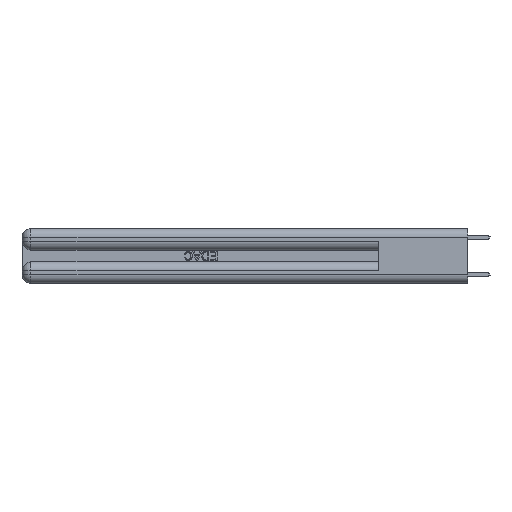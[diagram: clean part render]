
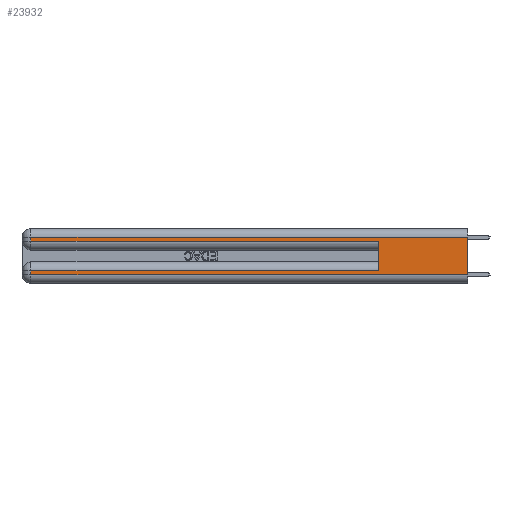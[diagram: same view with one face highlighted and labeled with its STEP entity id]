
A CAD part, left-side view. The second image highlights one B-rep face of the part: STEP entity #23932.
In plain terms, the highlighted planar face has unit normal (-1, 0, 0).
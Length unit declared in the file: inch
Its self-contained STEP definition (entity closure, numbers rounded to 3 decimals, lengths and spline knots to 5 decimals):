
#263 = LINE ( 'NONE', #33791, #25701 ) ;
#1139 = DIRECTION ( 'NONE',  ( 1., 0., 0. ) ) ;
#1954 = DIRECTION ( 'NONE',  ( 0., 0., -1. ) ) ;
#2128 = LINE ( 'NONE', #21906, #21447 ) ;
#2943 = DIRECTION ( 'NONE',  ( 0., 1., 0. ) ) ;
#3316 = VERTEX_POINT ( 'NONE', #34094 ) ;
#3340 = CARTESIAN_POINT ( 'NONE',  ( 0., 0., 0.37 ) ) ;
#3345 = VECTOR ( 'NONE', #18970, 39.37008 ) ;
#4038 = EDGE_CURVE ( 'NONE', #14277, #7153, #32106, .T. ) ;
#4164 = EDGE_CURVE ( 'NONE', #3316, #26474, #19611, .T. ) ;
#4542 = VECTOR ( 'NONE', #11597, 39.37008 ) ;
#4873 = CARTESIAN_POINT ( 'NONE',  ( 0., 2.94, 0.285 ) ) ;
#6800 = LINE ( 'NONE', #12837, #33855 ) ;
#7153 = VERTEX_POINT ( 'NONE', #12685 ) ;
#7225 = CARTESIAN_POINT ( 'NONE',  ( 0., 0., 0.085 ) ) ;
#8995 = ORIENTED_EDGE ( 'NONE', *, *, #10728, .T. ) ;
#9188 = VECTOR ( 'NONE', #35617, 39.37008 ) ;
#9305 = EDGE_LOOP ( 'NONE', ( #20092, #23945, #29942, #35041, #35452, #8995, #16218, #33614 ) ) ;
#10543 = CARTESIAN_POINT ( 'NONE',  ( 0., 0., 0.37 ) ) ;
#10728 = EDGE_CURVE ( 'NONE', #11101, #10753, #18948, .T. ) ;
#10753 = VERTEX_POINT ( 'NONE', #21346 ) ;
#10976 = EDGE_CURVE ( 'NONE', #26474, #23156, #17274, .T. ) ;
#11101 = VERTEX_POINT ( 'NONE', #29721 ) ;
#11597 = DIRECTION ( 'NONE',  ( 0., 0., -1. ) ) ;
#12053 = VERTEX_POINT ( 'NONE', #16623 ) ;
#12293 = FACE_OUTER_BOUND ( 'NONE', #9305, .T. ) ;
#12685 = CARTESIAN_POINT ( 'NONE',  ( 0., 0., 0.06 ) ) ;
#12837 = CARTESIAN_POINT ( 'NONE',  ( 0., 0., 0.285 ) ) ;
#12854 = CARTESIAN_POINT ( 'NONE',  ( 0., 0., 0.06 ) ) ;
#13350 = AXIS2_PLACEMENT_3D ( 'NONE', #3340, #1139, #33747 ) ;
#14277 = VERTEX_POINT ( 'NONE', #30823 ) ;
#14727 = DIRECTION ( 'NONE',  ( 0., 0., 1. ) ) ;
#15445 = VECTOR ( 'NONE', #2943, 39.37008 ) ;
#16042 = CARTESIAN_POINT ( 'NONE',  ( 0., 2.94, 0.31 ) ) ;
#16218 = ORIENTED_EDGE ( 'NONE', *, *, #32155, .T. ) ;
#16623 = CARTESIAN_POINT ( 'NONE',  ( 0., 0.6, 0.285 ) ) ;
#17274 = LINE ( 'NONE', #23135, #4542 ) ;
#18948 = LINE ( 'NONE', #7225, #9188 ) ;
#18970 = DIRECTION ( 'NONE',  ( 0., 0., -1. ) ) ;
#19611 = LINE ( 'NONE', #30781, #15445 ) ;
#20092 = ORIENTED_EDGE ( 'NONE', *, *, #31036, .F. ) ;
#21346 = CARTESIAN_POINT ( 'NONE',  ( 0., 2.94, 0.085 ) ) ;
#21447 = VECTOR ( 'NONE', #1954, 39.37008 ) ;
#21891 = VECTOR ( 'NONE', #27150, 39.37008 ) ;
#21906 = CARTESIAN_POINT ( 'NONE',  ( 0., 2.94, 0.37 ) ) ;
#23135 = CARTESIAN_POINT ( 'NONE',  ( 0., 2.94, 0.37 ) ) ;
#23156 = VERTEX_POINT ( 'NONE', #4873 ) ;
#23932 = ADVANCED_FACE ( 'NONE', ( #12293 ), #28815, .F. ) ;
#23945 = ORIENTED_EDGE ( 'NONE', *, *, #4164, .T. ) ;
#24023 = DIRECTION ( 'NONE',  ( 0., -1., 0. ) ) ;
#24066 = EDGE_CURVE ( 'NONE', #23156, #12053, #6800, .T. ) ;
#24827 = EDGE_CURVE ( 'NONE', #11101, #12053, #263, .T. ) ;
#25701 = VECTOR ( 'NONE', #14727, 39.37008 ) ;
#26474 = VERTEX_POINT ( 'NONE', #16042 ) ;
#27150 = DIRECTION ( 'NONE',  ( 0., -1., 0. ) ) ;
#28815 = PLANE ( 'NONE',  #13350 ) ;
#29427 = LINE ( 'NONE', #10543, #3345 ) ;
#29721 = CARTESIAN_POINT ( 'NONE',  ( 0., 0.6, 0.085 ) ) ;
#29942 = ORIENTED_EDGE ( 'NONE', *, *, #10976, .T. ) ;
#30781 = CARTESIAN_POINT ( 'NONE',  ( 0., 0., 0.31 ) ) ;
#30823 = CARTESIAN_POINT ( 'NONE',  ( 0., 2.94, 0.06 ) ) ;
#31036 = EDGE_CURVE ( 'NONE', #3316, #7153, #29427, .T. ) ;
#32106 = LINE ( 'NONE', #12854, #21891 ) ;
#32155 = EDGE_CURVE ( 'NONE', #10753, #14277, #2128, .T. ) ;
#33614 = ORIENTED_EDGE ( 'NONE', *, *, #4038, .T. ) ;
#33747 = DIRECTION ( 'NONE',  ( 0., 0., -1. ) ) ;
#33791 = CARTESIAN_POINT ( 'NONE',  ( 0., 0.6, 0.145 ) ) ;
#33855 = VECTOR ( 'NONE', #24023, 39.37008 ) ;
#34094 = CARTESIAN_POINT ( 'NONE',  ( 0., 0., 0.31 ) ) ;
#35041 = ORIENTED_EDGE ( 'NONE', *, *, #24066, .T. ) ;
#35452 = ORIENTED_EDGE ( 'NONE', *, *, #24827, .F. ) ;
#35617 = DIRECTION ( 'NONE',  ( 0., 1., 0. ) ) ;
